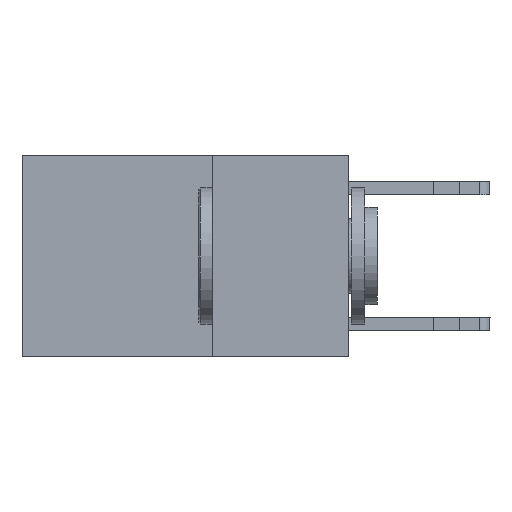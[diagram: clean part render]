
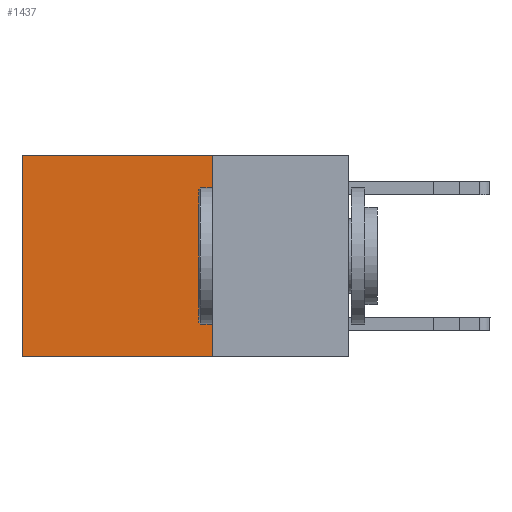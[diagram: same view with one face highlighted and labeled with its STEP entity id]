
A CAD part, left-side view. The second image highlights one B-rep face of the part: STEP entity #1437.
In plain terms, the highlighted planar face has unit normal (-1, 0, 0).
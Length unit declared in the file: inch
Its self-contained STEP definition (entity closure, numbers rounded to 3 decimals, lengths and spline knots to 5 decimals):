
#554 = CARTESIAN_POINT ( 'NONE',  ( 0.2625, 0.6, -0.37 ) ) ;
#1437 = ADVANCED_FACE ( 'NONE', ( #15510 ), #11433, .F. ) ;
#1603 = ORIENTED_EDGE ( 'NONE', *, *, #14926, .F. ) ;
#2107 = CARTESIAN_POINT ( 'NONE',  ( 0.2625, 0.6, 0. ) ) ;
#2625 = AXIS2_PLACEMENT_3D ( 'NONE', #11405, #11212, #11146 ) ;
#4423 = EDGE_CURVE ( 'NONE', #15917, #19014, #11430, .T. ) ;
#5049 = LINE ( 'NONE', #5221, #9534 ) ;
#5180 = ORIENTED_EDGE ( 'NONE', *, *, #4423, .T. ) ;
#5221 = CARTESIAN_POINT ( 'NONE',  ( 0.2625, 0.25, 0. ) ) ;
#5919 = VECTOR ( 'NONE', #10528, 39.37008 ) ;
#7104 = CARTESIAN_POINT ( 'NONE',  ( 0.2625, 0.25, 0. ) ) ;
#7185 = VERTEX_POINT ( 'NONE', #554 ) ;
#7351 = VECTOR ( 'NONE', #14640, 39.37008 ) ;
#7416 = EDGE_LOOP ( 'NONE', ( #12954, #12438, #1603, #5180 ) ) ;
#8374 = LINE ( 'NONE', #2107, #16976 ) ;
#8569 = CARTESIAN_POINT ( 'NONE',  ( 0.2625, 0.6, 0. ) ) ;
#8782 = CARTESIAN_POINT ( 'NONE',  ( 0.2625, 0.25, -0.37 ) ) ;
#9534 = VECTOR ( 'NONE', #11275, 39.37008 ) ;
#10528 = DIRECTION ( 'NONE',  ( 0., 1., 0. ) ) ;
#11146 = DIRECTION ( 'NONE',  ( 0., 0., -1. ) ) ;
#11212 = DIRECTION ( 'NONE',  ( 1., 0., 0. ) ) ;
#11275 = DIRECTION ( 'NONE',  ( 0., 0., -1. ) ) ;
#11317 = VERTEX_POINT ( 'NONE', #8782 ) ;
#11405 = CARTESIAN_POINT ( 'NONE',  ( 0.2625, 0.25, 0. ) ) ;
#11430 = LINE ( 'NONE', #17593, #7351 ) ;
#11433 = PLANE ( 'NONE',  #2625 ) ;
#12296 = EDGE_CURVE ( 'NONE', #19014, #7185, #8374, .T. ) ;
#12438 = ORIENTED_EDGE ( 'NONE', *, *, #17472, .F. ) ;
#12954 = ORIENTED_EDGE ( 'NONE', *, *, #12296, .T. ) ;
#13077 = LINE ( 'NONE', #19609, #5919 ) ;
#14640 = DIRECTION ( 'NONE',  ( 0., 1., 0. ) ) ;
#14926 = EDGE_CURVE ( 'NONE', #15917, #11317, #5049, .T. ) ;
#15510 = FACE_OUTER_BOUND ( 'NONE', #7416, .T. ) ;
#15917 = VERTEX_POINT ( 'NONE', #7104 ) ;
#16976 = VECTOR ( 'NONE', #18804, 39.37008 ) ;
#17472 = EDGE_CURVE ( 'NONE', #11317, #7185, #13077, .T. ) ;
#17593 = CARTESIAN_POINT ( 'NONE',  ( 0.2625, 0.25, 0. ) ) ;
#18804 = DIRECTION ( 'NONE',  ( 0., 0., -1. ) ) ;
#19014 = VERTEX_POINT ( 'NONE', #8569 ) ;
#19609 = CARTESIAN_POINT ( 'NONE',  ( 0.2625, 0.25, -0.37 ) ) ;
